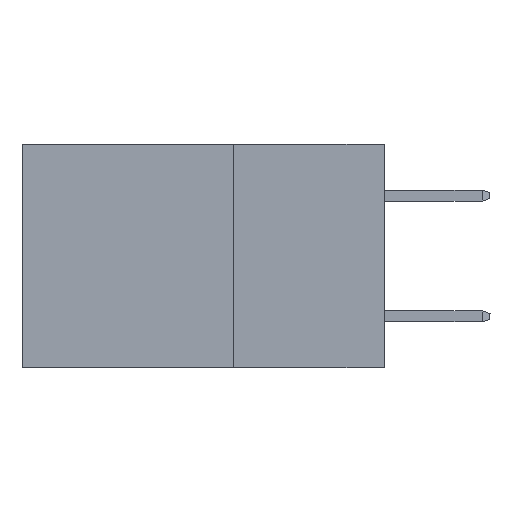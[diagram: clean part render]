
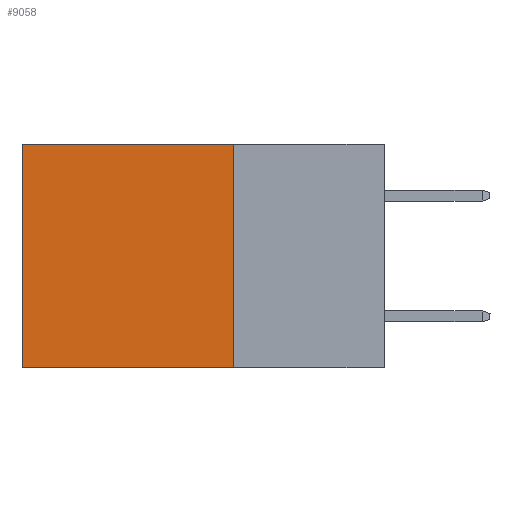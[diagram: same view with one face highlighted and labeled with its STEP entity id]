
A CAD part, left-side view. The second image highlights one B-rep face of the part: STEP entity #9058.
In plain terms, the highlighted planar face has unit normal (-1, 0, 0).
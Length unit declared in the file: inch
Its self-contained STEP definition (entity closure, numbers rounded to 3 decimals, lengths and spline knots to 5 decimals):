
#347 = DIRECTION ( 'NONE',  ( 0., 0., -1. ) ) ;
#966 = LINE ( 'NONE', #1691, #7770 ) ;
#1235 = VERTEX_POINT ( 'NONE', #7768 ) ;
#1553 = ORIENTED_EDGE ( 'NONE', *, *, #7155, .F. ) ;
#1678 = DIRECTION ( 'NONE',  ( 0., 0., -1. ) ) ;
#1691 = CARTESIAN_POINT ( 'NONE',  ( 0.2615, 0.6, -0.37 ) ) ;
#2203 = CARTESIAN_POINT ( 'NONE',  ( 0.2615, 0.6, -0.37 ) ) ;
#3379 = FACE_OUTER_BOUND ( 'NONE', #13234, .T. ) ;
#4285 = DIRECTION ( 'NONE',  ( 0., 1., 0. ) ) ;
#4345 = CARTESIAN_POINT ( 'NONE',  ( 0.2615, 0.25, 0. ) ) ;
#4667 = VECTOR ( 'NONE', #347, 39.37008 ) ;
#4907 = LINE ( 'NONE', #4345, #11324 ) ;
#5422 = CARTESIAN_POINT ( 'NONE',  ( 0.2615, 0.25, -0.37 ) ) ;
#5501 = LINE ( 'NONE', #10713, #14886 ) ;
#7155 = EDGE_CURVE ( 'NONE', #15869, #14297, #5501, .T. ) ;
#7768 = CARTESIAN_POINT ( 'NONE',  ( 0.2615, 0.25, 0. ) ) ;
#7770 = VECTOR ( 'NONE', #1678, 39.37008 ) ;
#8084 = LINE ( 'NONE', #5422, #4667 ) ;
#8282 = EDGE_CURVE ( 'NONE', #10742, #14297, #966, .T. ) ;
#9058 = ADVANCED_FACE ( 'NONE', ( #3379 ), #11787, .F. ) ;
#9384 = EDGE_CURVE ( 'NONE', #1235, #10742, #4907, .T. ) ;
#10129 = CARTESIAN_POINT ( 'NONE',  ( 0.2615, 0.6, 0. ) ) ;
#10695 = DIRECTION ( 'NONE',  ( 0., 1., 0. ) ) ;
#10713 = CARTESIAN_POINT ( 'NONE',  ( 0.2615, 0.25, -0.37 ) ) ;
#10742 = VERTEX_POINT ( 'NONE', #10129 ) ;
#11031 = DIRECTION ( 'NONE',  ( 0., 0., -1. ) ) ;
#11086 = DIRECTION ( 'NONE',  ( 1., 0., 0. ) ) ;
#11123 = CARTESIAN_POINT ( 'NONE',  ( 0.2615, 0.25, -0.37 ) ) ;
#11324 = VECTOR ( 'NONE', #4285, 39.37008 ) ;
#11423 = ORIENTED_EDGE ( 'NONE', *, *, #9384, .T. ) ;
#11623 = CARTESIAN_POINT ( 'NONE',  ( 0.2615, 0.25, -0.37 ) ) ;
#11787 = PLANE ( 'NONE',  #15056 ) ;
#13234 = EDGE_LOOP ( 'NONE', ( #14965, #1553, #15115, #11423 ) ) ;
#14297 = VERTEX_POINT ( 'NONE', #2203 ) ;
#14886 = VECTOR ( 'NONE', #10695, 39.37008 ) ;
#14965 = ORIENTED_EDGE ( 'NONE', *, *, #8282, .T. ) ;
#15056 = AXIS2_PLACEMENT_3D ( 'NONE', #11123, #11086, #11031 ) ;
#15115 = ORIENTED_EDGE ( 'NONE', *, *, #15367, .F. ) ;
#15367 = EDGE_CURVE ( 'NONE', #1235, #15869, #8084, .T. ) ;
#15869 = VERTEX_POINT ( 'NONE', #11623 ) ;
